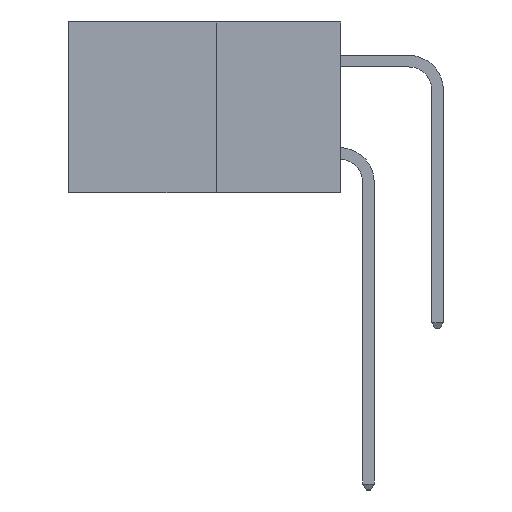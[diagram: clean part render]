
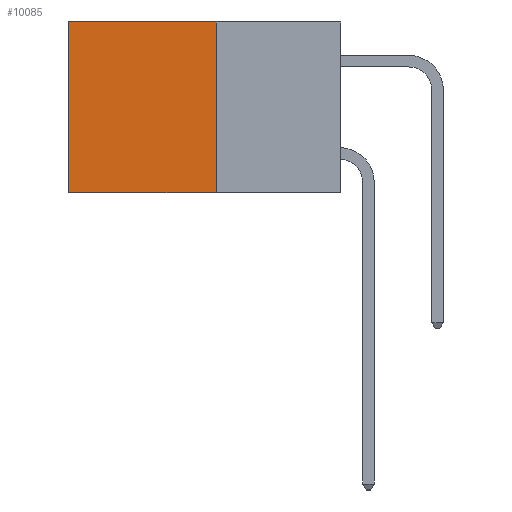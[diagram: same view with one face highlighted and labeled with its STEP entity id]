
A CAD part, left-side view. The second image highlights one B-rep face of the part: STEP entity #10085.
In plain terms, the highlighted planar face has unit normal (-1, 0, 0).
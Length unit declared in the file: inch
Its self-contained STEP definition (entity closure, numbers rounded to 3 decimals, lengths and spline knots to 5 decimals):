
#106 = CARTESIAN_POINT ( 'NONE',  ( 0.277, 0.27, -0.37 ) ) ;
#296 = LINE ( 'NONE', #7770, #10692 ) ;
#554 = EDGE_CURVE ( 'NONE', #12576, #11360, #16841, .T. ) ;
#956 = CARTESIAN_POINT ( 'NONE',  ( 0.277, 0.27, 0. ) ) ;
#1999 = CARTESIAN_POINT ( 'NONE',  ( 0.277, 0.59, 0. ) ) ;
#2236 = DIRECTION ( 'NONE',  ( 0., 1., 0. ) ) ;
#4277 = LINE ( 'NONE', #18906, #15913 ) ;
#4671 = CARTESIAN_POINT ( 'NONE',  ( 0.277, 0.59, -0.37 ) ) ;
#5041 = PLANE ( 'NONE',  #15630 ) ;
#7770 = CARTESIAN_POINT ( 'NONE',  ( 0.277, 0.27, 0. ) ) ;
#8009 = DIRECTION ( 'NONE',  ( 1., 0., 0. ) ) ;
#9211 = FACE_OUTER_BOUND ( 'NONE', #10253, .T. ) ;
#10085 = ADVANCED_FACE ( 'NONE', ( #9211 ), #5041, .F. ) ;
#10142 = DIRECTION ( 'NONE',  ( 0., 0., -1. ) ) ;
#10253 = EDGE_LOOP ( 'NONE', ( #10402, #11596, #12012, #12449 ) ) ;
#10402 = ORIENTED_EDGE ( 'NONE', *, *, #13127, .T. ) ;
#10692 = VECTOR ( 'NONE', #16549, 39.37008 ) ;
#10922 = LINE ( 'NONE', #18928, #18238 ) ;
#11360 = VERTEX_POINT ( 'NONE', #4671 ) ;
#11596 = ORIENTED_EDGE ( 'NONE', *, *, #554, .F. ) ;
#11622 = DIRECTION ( 'NONE',  ( 0., 0., -1. ) ) ;
#11838 = CARTESIAN_POINT ( 'NONE',  ( 0.277, 0.27, -0.37 ) ) ;
#12012 = ORIENTED_EDGE ( 'NONE', *, *, #13750, .F. ) ;
#12449 = ORIENTED_EDGE ( 'NONE', *, *, #13355, .T. ) ;
#12576 = VERTEX_POINT ( 'NONE', #106 ) ;
#12961 = VECTOR ( 'NONE', #2236, 39.37008 ) ;
#13127 = EDGE_CURVE ( 'NONE', #16730, #11360, #10922, .T. ) ;
#13355 = EDGE_CURVE ( 'NONE', #17873, #16730, #296, .T. ) ;
#13750 = EDGE_CURVE ( 'NONE', #17873, #12576, #4277, .T. ) ;
#15630 = AXIS2_PLACEMENT_3D ( 'NONE', #16720, #8009, #18197 ) ;
#15913 = VECTOR ( 'NONE', #10142, 39.37008 ) ;
#16549 = DIRECTION ( 'NONE',  ( 0., 1., 0. ) ) ;
#16720 = CARTESIAN_POINT ( 'NONE',  ( 0.277, 0.27, -0.37 ) ) ;
#16730 = VERTEX_POINT ( 'NONE', #1999 ) ;
#16841 = LINE ( 'NONE', #11838, #12961 ) ;
#17873 = VERTEX_POINT ( 'NONE', #956 ) ;
#18197 = DIRECTION ( 'NONE',  ( 0., 0., -1. ) ) ;
#18238 = VECTOR ( 'NONE', #11622, 39.37008 ) ;
#18906 = CARTESIAN_POINT ( 'NONE',  ( 0.277, 0.27, -0.37 ) ) ;
#18928 = CARTESIAN_POINT ( 'NONE',  ( 0.277, 0.59, -0.37 ) ) ;
